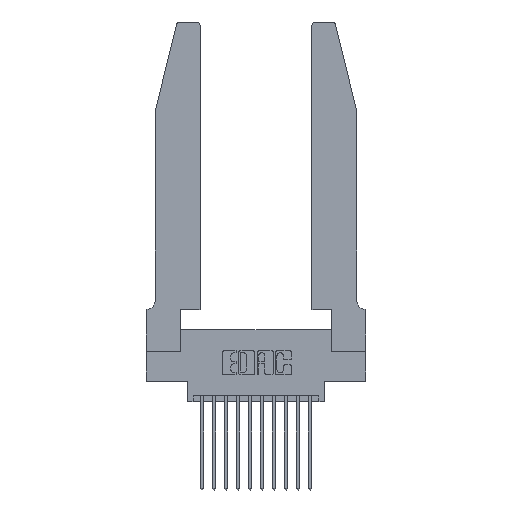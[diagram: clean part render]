
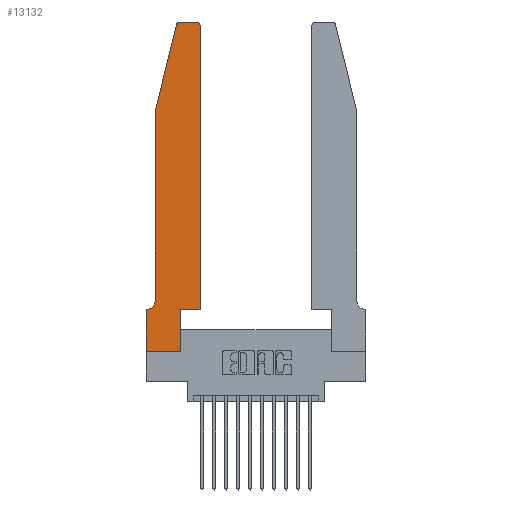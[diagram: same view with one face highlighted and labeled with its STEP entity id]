
A CAD part, top view. The second image highlights one B-rep face of the part: STEP entity #13132.
In plain terms, the highlighted planar face has unit normal (0, 0, 1).
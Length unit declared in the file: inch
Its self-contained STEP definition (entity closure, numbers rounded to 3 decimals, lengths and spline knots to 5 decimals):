
#360 = EDGE_CURVE ( 'NONE', #4595, #5387, #6024, .T. ) ;
#440 = VERTEX_POINT ( 'NONE', #12630 ) ;
#584 = EDGE_CURVE ( 'NONE', #440, #11891, #10138, .T. ) ;
#662 = CARTESIAN_POINT ( 'NONE',  ( 0.0755, 0.42, 0.37 ) ) ;
#686 = DIRECTION ( 'NONE',  ( -1., 0., 0. ) ) ;
#758 = LINE ( 'NONE', #9177, #4304 ) ;
#855 = ORIENTED_EDGE ( 'NONE', *, *, #9923, .T. ) ;
#1390 = LINE ( 'NONE', #8632, #4951 ) ;
#1555 = EDGE_CURVE ( 'NONE', #12193, #4595, #6845, .T. ) ;
#1556 = VECTOR ( 'NONE', #9479, 39.37008 ) ;
#1719 = VERTEX_POINT ( 'NONE', #10260 ) ;
#1887 = ORIENTED_EDGE ( 'NONE', *, *, #584, .T. ) ;
#1994 = DIRECTION ( 'NONE',  ( 1., 0., 0. ) ) ;
#2081 = LINE ( 'NONE', #7157, #12224 ) ;
#2374 = VERTEX_POINT ( 'NONE', #14864 ) ;
#2635 = CARTESIAN_POINT ( 'NONE',  ( 0.25487, 2.72718, 0.37 ) ) ;
#2704 = AXIS2_PLACEMENT_3D ( 'NONE', #16482, #8686, #686 ) ;
#2716 = VECTOR ( 'NONE', #11826, 39.37008 ) ;
#2734 = ORIENTED_EDGE ( 'NONE', *, *, #1555, .T. ) ;
#2779 = VECTOR ( 'NONE', #5487, 39.37008 ) ;
#2945 = AXIS2_PLACEMENT_3D ( 'NONE', #14521, #9253, #11948 ) ;
#3696 = ORIENTED_EDGE ( 'NONE', *, *, #12648, .T. ) ;
#3712 = EDGE_CURVE ( 'NONE', #11891, #2374, #12137, .T. ) ;
#4095 = CARTESIAN_POINT ( 'NONE',  ( 0.0755, 2., 0.37 ) ) ;
#4304 = VECTOR ( 'NONE', #16966, 39.37008 ) ;
#4595 = VERTEX_POINT ( 'NONE', #7416 ) ;
#4897 = CARTESIAN_POINT ( 'NONE',  ( 0.0755, 2., 0.37 ) ) ;
#4951 = VECTOR ( 'NONE', #1994, 39.37008 ) ;
#5354 = CARTESIAN_POINT ( 'NONE',  ( 0.4205, 2.75, 0.37 ) ) ;
#5387 = VERTEX_POINT ( 'NONE', #14876 ) ;
#5487 = DIRECTION ( 'NONE',  ( 0., -1., 0. ) ) ;
#6014 = ORIENTED_EDGE ( 'NONE', *, *, #360, .T. ) ;
#6024 = LINE ( 'NONE', #9130, #9146 ) ;
#6257 = LINE ( 'NONE', #13149, #2716 ) ;
#6845 = LINE ( 'NONE', #7333, #7290 ) ;
#7157 = CARTESIAN_POINT ( 'NONE',  ( 0.4505, 0.35, 0.37 ) ) ;
#7208 = CARTESIAN_POINT ( 'NONE',  ( 0.4205, 2.72, 0.37 ) ) ;
#7290 = VECTOR ( 'NONE', #8301, 39.37008 ) ;
#7333 = CARTESIAN_POINT ( 'NONE',  ( 0.0755, 0.35, 0.37 ) ) ;
#7416 = CARTESIAN_POINT ( 'NONE',  ( 0., 0.35, 0.37 ) ) ;
#7523 = CIRCLE ( 'NONE', #2704, 0.07 ) ;
#7786 = CARTESIAN_POINT ( 'NONE',  ( 0.284, 2.72, 0.37 ) ) ;
#7813 = ORIENTED_EDGE ( 'NONE', *, *, #10508, .T. ) ;
#7994 = CIRCLE ( 'NONE', #8640, 0.03 ) ;
#8017 = EDGE_LOOP ( 'NONE', ( #16608, #9085, #11021, #3696, #855, #2734, #6014, #14317, #12192, #8277, #7813, #1887 ) ) ;
#8170 = CARTESIAN_POINT ( 'NONE',  ( 0.2605, 2.75, 0.37 ) ) ;
#8242 = VERTEX_POINT ( 'NONE', #13784 ) ;
#8277 = ORIENTED_EDGE ( 'NONE', *, *, #16267, .T. ) ;
#8301 = DIRECTION ( 'NONE',  ( -1., 0., 0. ) ) ;
#8601 = CARTESIAN_POINT ( 'NONE',  ( 0.0055, 0.35, 0.37 ) ) ;
#8632 = CARTESIAN_POINT ( 'NONE',  ( 0., 0., 0.37 ) ) ;
#8640 = AXIS2_PLACEMENT_3D ( 'NONE', #7786, #16876, #9083 ) ;
#8686 = DIRECTION ( 'NONE',  ( 0., 0., -1. ) ) ;
#9083 = DIRECTION ( 'NONE',  ( 1., 0., 0. ) ) ;
#9085 = ORIENTED_EDGE ( 'NONE', *, *, #13015, .T. ) ;
#9130 = CARTESIAN_POINT ( 'NONE',  ( 0., 0., 0.37 ) ) ;
#9146 = VECTOR ( 'NONE', #10807, 39.37008 ) ;
#9177 = CARTESIAN_POINT ( 'NONE',  ( 0.2865, 0.35, 0.37 ) ) ;
#9195 = DIRECTION ( 'NONE',  ( 1., 0., 0. ) ) ;
#9253 = DIRECTION ( 'NONE',  ( 0., 0., 1. ) ) ;
#9260 = DIRECTION ( 'NONE',  ( 1., 0., 0. ) ) ;
#9316 = PLANE ( 'NONE',  #2945 ) ;
#9479 = DIRECTION ( 'NONE',  ( -1., 0., 0. ) ) ;
#9806 = FACE_OUTER_BOUND ( 'NONE', #8017, .T. ) ;
#9923 = EDGE_CURVE ( 'NONE', #12228, #12193, #7523, .T. ) ;
#10138 = CIRCLE ( 'NONE', #10462, 0.03 ) ;
#10242 = EDGE_CURVE ( 'NONE', #14689, #11664, #6257, .T. ) ;
#10260 = CARTESIAN_POINT ( 'NONE',  ( 0.2865, 0.35, 0.37 ) ) ;
#10462 = AXIS2_PLACEMENT_3D ( 'NONE', #7208, #13453, #9260 ) ;
#10508 = EDGE_CURVE ( 'NONE', #8242, #440, #2081, .T. ) ;
#10807 = DIRECTION ( 'NONE',  ( 0., -1., 0. ) ) ;
#11021 = ORIENTED_EDGE ( 'NONE', *, *, #10242, .T. ) ;
#11575 = LINE ( 'NONE', #11774, #14641 ) ;
#11664 = VERTEX_POINT ( 'NONE', #4897 ) ;
#11774 = CARTESIAN_POINT ( 'NONE',  ( 0.4505, 0.35, 0.37 ) ) ;
#11826 = DIRECTION ( 'NONE',  ( -0.239, -0.971, 0. ) ) ;
#11891 = VERTEX_POINT ( 'NONE', #5354 ) ;
#11948 = DIRECTION ( 'NONE',  ( 1., 0., 0. ) ) ;
#12137 = LINE ( 'NONE', #8170, #1556 ) ;
#12192 = ORIENTED_EDGE ( 'NONE', *, *, #17007, .T. ) ;
#12193 = VERTEX_POINT ( 'NONE', #8601 ) ;
#12224 = VECTOR ( 'NONE', #14989, 39.37008 ) ;
#12228 = VERTEX_POINT ( 'NONE', #662 ) ;
#12630 = CARTESIAN_POINT ( 'NONE',  ( 0.4505, 2.72, 0.37 ) ) ;
#12648 = EDGE_CURVE ( 'NONE', #11664, #12228, #13328, .T. ) ;
#13015 = EDGE_CURVE ( 'NONE', #2374, #14689, #7994, .T. ) ;
#13132 = ADVANCED_FACE ( 'NONE', ( #9806 ), #9316, .T. ) ;
#13149 = CARTESIAN_POINT ( 'NONE',  ( 0.0755, 2., 0.37 ) ) ;
#13328 = LINE ( 'NONE', #4095, #2779 ) ;
#13453 = DIRECTION ( 'NONE',  ( 0., 0., 1. ) ) ;
#13784 = CARTESIAN_POINT ( 'NONE',  ( 0.4505, 0.35, 0.37 ) ) ;
#14317 = ORIENTED_EDGE ( 'NONE', *, *, #16026, .T. ) ;
#14521 = CARTESIAN_POINT ( 'NONE',  ( 0., 0.35, 0.37 ) ) ;
#14641 = VECTOR ( 'NONE', #9195, 39.37008 ) ;
#14689 = VERTEX_POINT ( 'NONE', #2635 ) ;
#14864 = CARTESIAN_POINT ( 'NONE',  ( 0.284, 2.75, 0.37 ) ) ;
#14876 = CARTESIAN_POINT ( 'NONE',  ( 0., 0., 0.37 ) ) ;
#14989 = DIRECTION ( 'NONE',  ( 0., 1., 0. ) ) ;
#15591 = CARTESIAN_POINT ( 'NONE',  ( 0.2865, 0., 0.37 ) ) ;
#15621 = VERTEX_POINT ( 'NONE', #15591 ) ;
#16026 = EDGE_CURVE ( 'NONE', #5387, #15621, #1390, .T. ) ;
#16267 = EDGE_CURVE ( 'NONE', #1719, #8242, #11575, .T. ) ;
#16482 = CARTESIAN_POINT ( 'NONE',  ( 0.0055, 0.42, 0.37 ) ) ;
#16608 = ORIENTED_EDGE ( 'NONE', *, *, #3712, .T. ) ;
#16876 = DIRECTION ( 'NONE',  ( 0., 0., 1. ) ) ;
#16966 = DIRECTION ( 'NONE',  ( 0., 1., 0. ) ) ;
#17007 = EDGE_CURVE ( 'NONE', #15621, #1719, #758, .T. ) ;
